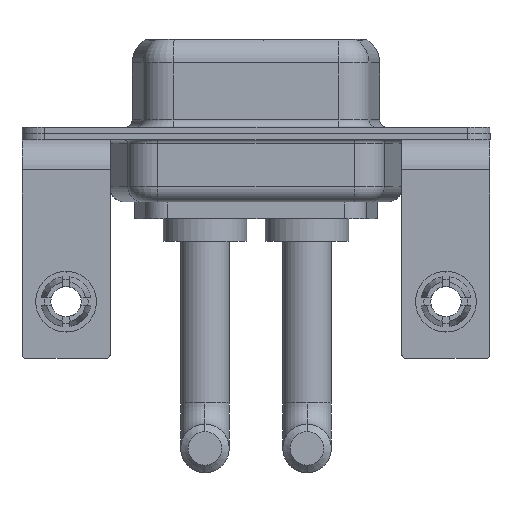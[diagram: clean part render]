
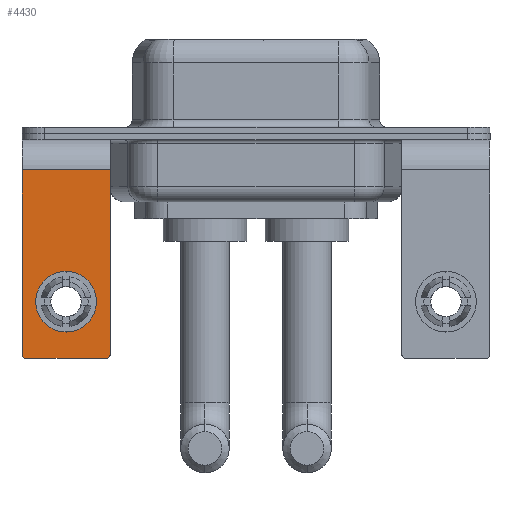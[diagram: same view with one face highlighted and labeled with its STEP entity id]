
A CAD part, front view. The second image highlights one B-rep face of the part: STEP entity #4430.
In plain terms, the highlighted planar face has unit normal (0, -1, 0).
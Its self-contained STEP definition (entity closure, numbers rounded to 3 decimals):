
#167 = EDGE_CURVE ( 'NONE', #5516, #4710, #6174, .T. ) ;
#399 = EDGE_CURVE ( 'NONE', #4710, #5516, #5117, .T. ) ;
#533 = CARTESIAN_POINT ( 'NONE',  ( -2.9, -6.25, -2.4 ) ) ;
#931 = DIRECTION ( 'NONE',  ( 0., 0., -1. ) ) ;
#1037 = DIRECTION ( 'NONE',  ( -1., 0., 0. ) ) ;
#1101 = VERTEX_POINT ( 'NONE', #13789 ) ;
#1670 = DIRECTION ( 'NONE',  ( 0., 0., 1. ) ) ;
#1829 = EDGE_CURVE ( 'NONE', #1101, #10567, #3623, .T. ) ;
#2223 = CARTESIAN_POINT ( 'NONE',  ( 2.65, -6.25, -14.55 ) ) ;
#2271 = EDGE_CURVE ( 'NONE', #14008, #12956, #10289, .T. ) ;
#2348 = DIRECTION ( 'NONE',  ( 0., 0., -1. ) ) ;
#2461 = LINE ( 'NONE', #13518, #3981 ) ;
#3056 = EDGE_CURVE ( 'NONE', #15621, #14008, #11926, .T. ) ;
#3623 = LINE ( 'NONE', #9599, #8999 ) ;
#3981 = VECTOR ( 'NONE', #7394, 1000. ) ;
#4371 = FACE_OUTER_BOUND ( 'NONE', #10681, .T. ) ;
#4430 = ADVANCED_FACE ( 'NONE', ( #11469, #4371 ), #15334, .F. ) ;
#4493 = ORIENTED_EDGE ( 'NONE', *, *, #4532, .T. ) ;
#4532 = EDGE_CURVE ( 'NONE', #7538, #10567, #5835, .T. ) ;
#4710 = VERTEX_POINT ( 'NONE', #10015 ) ;
#4772 = DIRECTION ( 'NONE',  ( 0., -1., 0. ) ) ;
#4783 = ORIENTED_EDGE ( 'NONE', *, *, #1829, .F. ) ;
#5117 = CIRCLE ( 'NONE', #13989, 2. ) ;
#5502 = CARTESIAN_POINT ( 'NONE',  ( 2.9, -6.25, -14.55 ) ) ;
#5516 = VERTEX_POINT ( 'NONE', #14758 ) ;
#5781 = ORIENTED_EDGE ( 'NONE', *, *, #2271, .T. ) ;
#5784 = CARTESIAN_POINT ( 'NONE',  ( -2.9, -6.25, -2.4 ) ) ;
#5835 = CIRCLE ( 'NONE', #6850, 0.25 ) ;
#5889 = CARTESIAN_POINT ( 'NONE',  ( 0., -6.25, -11.07 ) ) ;
#6041 = DIRECTION ( 'NONE',  ( 0., 0., 1. ) ) ;
#6129 = CARTESIAN_POINT ( 'NONE',  ( 0., -6.25, -11.07 ) ) ;
#6174 = CIRCLE ( 'NONE', #8199, 2. ) ;
#6495 = EDGE_LOOP ( 'NONE', ( #9291, #9169 ) ) ;
#6550 = DIRECTION ( 'NONE',  ( 0., -1., 0. ) ) ;
#6850 = AXIS2_PLACEMENT_3D ( 'NONE', #2223, #4772, #6041 ) ;
#6950 = ORIENTED_EDGE ( 'NONE', *, *, #3056, .T. ) ;
#7280 = VECTOR ( 'NONE', #1037, 1000. ) ;
#7394 = DIRECTION ( 'NONE',  ( -1., 0., 0. ) ) ;
#7538 = VERTEX_POINT ( 'NONE', #8788 ) ;
#8102 = CARTESIAN_POINT ( 'NONE',  ( 2.9, -6.25, -2.4 ) ) ;
#8197 = DIRECTION ( 'NONE',  ( 0., 0., 1. ) ) ;
#8199 = AXIS2_PLACEMENT_3D ( 'NONE', #5889, #9246, #8197 ) ;
#8788 = CARTESIAN_POINT ( 'NONE',  ( 2.65, -6.25, -14.8 ) ) ;
#8964 = ORIENTED_EDGE ( 'NONE', *, *, #14681, .F. ) ;
#8986 = CARTESIAN_POINT ( 'NONE',  ( -2.65, -6.25, -14.8 ) ) ;
#8999 = VECTOR ( 'NONE', #2348, 1000. ) ;
#9169 = ORIENTED_EDGE ( 'NONE', *, *, #167, .T. ) ;
#9246 = DIRECTION ( 'NONE',  ( 0., 1., 0. ) ) ;
#9265 = CARTESIAN_POINT ( 'NONE',  ( -2.65, -6.25, -14.55 ) ) ;
#9291 = ORIENTED_EDGE ( 'NONE', *, *, #399, .T. ) ;
#9599 = CARTESIAN_POINT ( 'NONE',  ( 2.9, -6.25, -2.4 ) ) ;
#9799 = DIRECTION ( 'NONE',  ( 0., 1., 0. ) ) ;
#10015 = CARTESIAN_POINT ( 'NONE',  ( 0., -6.25, -13.07 ) ) ;
#10289 = CIRCLE ( 'NONE', #14599, 0.25 ) ;
#10567 = VERTEX_POINT ( 'NONE', #5502 ) ;
#10587 = DIRECTION ( 'NONE',  ( 0., 0., 1. ) ) ;
#10681 = EDGE_LOOP ( 'NONE', ( #6950, #5781, #8964, #4493, #4783, #15470 ) ) ;
#11469 = FACE_BOUND ( 'NONE', #6495, .T. ) ;
#11926 = LINE ( 'NONE', #5784, #12533 ) ;
#12106 = CARTESIAN_POINT ( 'NONE',  ( 2.9, -6.25, -2.4 ) ) ;
#12533 = VECTOR ( 'NONE', #931, 1000. ) ;
#12956 = VERTEX_POINT ( 'NONE', #8986 ) ;
#13518 = CARTESIAN_POINT ( 'NONE',  ( 2.9, -6.25, -14.8 ) ) ;
#13712 = AXIS2_PLACEMENT_3D ( 'NONE', #8102, #15175, #10587 ) ;
#13789 = CARTESIAN_POINT ( 'NONE',  ( 2.9, -6.25, -2.4 ) ) ;
#13989 = AXIS2_PLACEMENT_3D ( 'NONE', #6129, #9799, #1670 ) ;
#14008 = VERTEX_POINT ( 'NONE', #14030 ) ;
#14030 = CARTESIAN_POINT ( 'NONE',  ( -2.9, -6.25, -14.55 ) ) ;
#14112 = DIRECTION ( 'NONE',  ( 0., 0., 1. ) ) ;
#14599 = AXIS2_PLACEMENT_3D ( 'NONE', #9265, #6550, #14112 ) ;
#14603 = EDGE_CURVE ( 'NONE', #1101, #15621, #15662, .T. ) ;
#14681 = EDGE_CURVE ( 'NONE', #7538, #12956, #2461, .T. ) ;
#14758 = CARTESIAN_POINT ( 'NONE',  ( 0., -6.25, -9.07 ) ) ;
#15175 = DIRECTION ( 'NONE',  ( 0., 1., 0. ) ) ;
#15334 = PLANE ( 'NONE',  #13712 ) ;
#15470 = ORIENTED_EDGE ( 'NONE', *, *, #14603, .T. ) ;
#15621 = VERTEX_POINT ( 'NONE', #533 ) ;
#15662 = LINE ( 'NONE', #12106, #7280 ) ;
